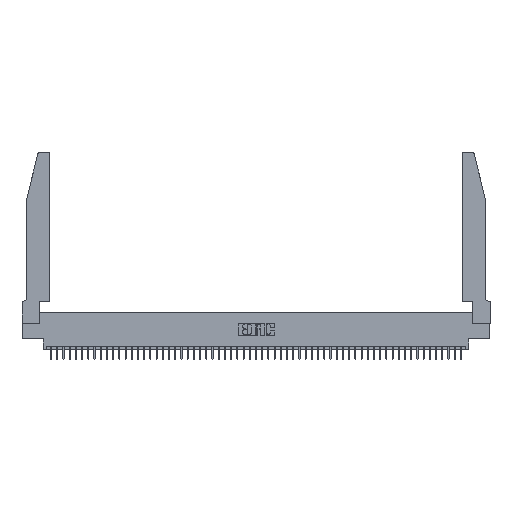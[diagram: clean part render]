
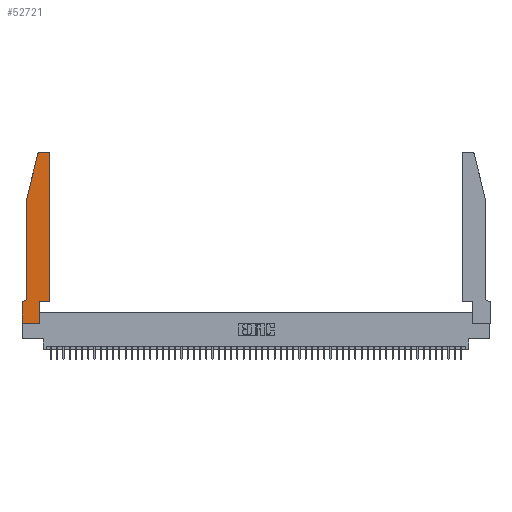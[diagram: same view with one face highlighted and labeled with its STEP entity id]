
A CAD part, top view. The second image highlights one B-rep face of the part: STEP entity #52721.
In plain terms, the highlighted planar face has unit normal (0, 0, 1).
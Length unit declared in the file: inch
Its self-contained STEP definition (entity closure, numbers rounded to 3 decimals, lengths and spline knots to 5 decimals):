
#729 = DIRECTION ( 'NONE',  ( 1., 0., 0. ) ) ;
#968 = VECTOR ( 'NONE', #33192, 39.37008 ) ;
#1160 = EDGE_CURVE ( 'NONE', #38254, #40192, #9611, .T. ) ;
#1197 = CARTESIAN_POINT ( 'NONE',  ( 0.4205, 2.72, 0.37 ) ) ;
#1478 = LINE ( 'NONE', #21008, #22473 ) ;
#1681 = LINE ( 'NONE', #25852, #3002 ) ;
#1808 = ORIENTED_EDGE ( 'NONE', *, *, #1160, .T. ) ;
#2245 = VERTEX_POINT ( 'NONE', #37265 ) ;
#2338 = DIRECTION ( 'NONE',  ( 0., 0., 1. ) ) ;
#2991 = CARTESIAN_POINT ( 'NONE',  ( 0.0055, 0.35, 0.37 ) ) ;
#3002 = VECTOR ( 'NONE', #729, 39.37008 ) ;
#3224 = ORIENTED_EDGE ( 'NONE', *, *, #48681, .T. ) ;
#4009 = CARTESIAN_POINT ( 'NONE',  ( 0.4205, 2.75, 0.37 ) ) ;
#5433 = DIRECTION ( 'NONE',  ( 1., 0., 0. ) ) ;
#7409 = ORIENTED_EDGE ( 'NONE', *, *, #41785, .T. ) ;
#7880 = CARTESIAN_POINT ( 'NONE',  ( 0., 0., 0.37 ) ) ;
#8603 = CARTESIAN_POINT ( 'NONE',  ( 0.4505, 2.72, 0.37 ) ) ;
#9611 = CIRCLE ( 'NONE', #31073, 0.03 ) ;
#10171 = VERTEX_POINT ( 'NONE', #50380 ) ;
#10530 = LINE ( 'NONE', #48544, #42684 ) ;
#10704 = CARTESIAN_POINT ( 'NONE',  ( 0.2865, 0., 0.37 ) ) ;
#10878 = DIRECTION ( 'NONE',  ( 0., 0., -1. ) ) ;
#11372 = CARTESIAN_POINT ( 'NONE',  ( 0., 0.35, 0.37 ) ) ;
#12225 = ORIENTED_EDGE ( 'NONE', *, *, #20809, .T. ) ;
#13235 = VERTEX_POINT ( 'NONE', #36837 ) ;
#14079 = ORIENTED_EDGE ( 'NONE', *, *, #31133, .T. ) ;
#14573 = VERTEX_POINT ( 'NONE', #11372 ) ;
#15166 = ORIENTED_EDGE ( 'NONE', *, *, #44168, .T. ) ;
#15667 = VERTEX_POINT ( 'NONE', #17763 ) ;
#15708 = VECTOR ( 'NONE', #51300, 39.37008 ) ;
#16157 = ORIENTED_EDGE ( 'NONE', *, *, #49384, .T. ) ;
#16404 = AXIS2_PLACEMENT_3D ( 'NONE', #36039, #10878, #40196 ) ;
#16542 = EDGE_CURVE ( 'NONE', #13235, #23261, #33527, .T. ) ;
#16600 = DIRECTION ( 'NONE',  ( -0.239, -0.971, 0. ) ) ;
#17763 = CARTESIAN_POINT ( 'NONE',  ( 0.25487, 2.72718, 0.37 ) ) ;
#17902 = CARTESIAN_POINT ( 'NONE',  ( 0.2605, 2.75, 0.37 ) ) ;
#17969 = VERTEX_POINT ( 'NONE', #10704 ) ;
#19285 = CARTESIAN_POINT ( 'NONE',  ( 0.2865, 0.35, 0.37 ) ) ;
#19625 = FACE_OUTER_BOUND ( 'NONE', #51829, .T. ) ;
#20610 = CARTESIAN_POINT ( 'NONE',  ( 0.0755, 2., 0.37 ) ) ;
#20809 = EDGE_CURVE ( 'NONE', #43978, #13235, #1478, .T. ) ;
#21008 = CARTESIAN_POINT ( 'NONE',  ( 0.0755, 2., 0.37 ) ) ;
#21282 = ORIENTED_EDGE ( 'NONE', *, *, #43305, .T. ) ;
#22114 = PLANE ( 'NONE',  #34845 ) ;
#22290 = CARTESIAN_POINT ( 'NONE',  ( 0., 0.35, 0.37 ) ) ;
#22473 = VECTOR ( 'NONE', #35866, 39.37008 ) ;
#23261 = VERTEX_POINT ( 'NONE', #2991 ) ;
#23272 = LINE ( 'NONE', #28945, #968 ) ;
#23498 = DIRECTION ( 'NONE',  ( 0., 1., 0. ) ) ;
#23555 = DIRECTION ( 'NONE',  ( 0., 1., 0. ) ) ;
#25852 = CARTESIAN_POINT ( 'NONE',  ( 0.4505, 0.35, 0.37 ) ) ;
#26543 = DIRECTION ( 'NONE',  ( 1., 0., 0. ) ) ;
#27492 = CARTESIAN_POINT ( 'NONE',  ( 0.284, 2.72, 0.37 ) ) ;
#27785 = CARTESIAN_POINT ( 'NONE',  ( 0.4505, 0.35, 0.37 ) ) ;
#28052 = VECTOR ( 'NONE', #44720, 39.37008 ) ;
#28945 = CARTESIAN_POINT ( 'NONE',  ( 0., 0., 0.37 ) ) ;
#30451 = EDGE_CURVE ( 'NONE', #17969, #2245, #31289, .T. ) ;
#30556 = DIRECTION ( 'NONE',  ( 0., 0., 1. ) ) ;
#30857 = EDGE_CURVE ( 'NONE', #2245, #10171, #1681, .T. ) ;
#31073 = AXIS2_PLACEMENT_3D ( 'NONE', #1197, #30556, #5433 ) ;
#31084 = VECTOR ( 'NONE', #16600, 39.37008 ) ;
#31133 = EDGE_CURVE ( 'NONE', #49515, #15667, #54010, .T. ) ;
#31289 = LINE ( 'NONE', #19285, #52131 ) ;
#31714 = DIRECTION ( 'NONE',  ( 1., 0., 0. ) ) ;
#31784 = LINE ( 'NONE', #27785, #52614 ) ;
#33192 = DIRECTION ( 'NONE',  ( 1., 0., 0. ) ) ;
#33527 = CIRCLE ( 'NONE', #16404, 0.07 ) ;
#34845 = AXIS2_PLACEMENT_3D ( 'NONE', #22290, #51516, #26543 ) ;
#35866 = DIRECTION ( 'NONE',  ( 0., -1., 0. ) ) ;
#36008 = DIRECTION ( 'NONE',  ( -1., 0., 0. ) ) ;
#36039 = CARTESIAN_POINT ( 'NONE',  ( 0.0055, 0.42, 0.37 ) ) ;
#36837 = CARTESIAN_POINT ( 'NONE',  ( 0.0755, 0.42, 0.37 ) ) ;
#37265 = CARTESIAN_POINT ( 'NONE',  ( 0.2865, 0.35, 0.37 ) ) ;
#38026 = LINE ( 'NONE', #17902, #15708 ) ;
#38231 = CARTESIAN_POINT ( 'NONE',  ( 0.284, 2.75, 0.37 ) ) ;
#38254 = VERTEX_POINT ( 'NONE', #8603 ) ;
#40192 = VERTEX_POINT ( 'NONE', #4009 ) ;
#40196 = DIRECTION ( 'NONE',  ( -1., 0., 0. ) ) ;
#40520 = CARTESIAN_POINT ( 'NONE',  ( 0., 0., 0.37 ) ) ;
#41785 = EDGE_CURVE ( 'NONE', #23261, #14573, #10530, .T. ) ;
#41856 = LINE ( 'NONE', #40520, #28052 ) ;
#42498 = VERTEX_POINT ( 'NONE', #7880 ) ;
#42684 = VECTOR ( 'NONE', #36008, 39.37008 ) ;
#43305 = EDGE_CURVE ( 'NONE', #40192, #49515, #38026, .T. ) ;
#43978 = VERTEX_POINT ( 'NONE', #47462 ) ;
#44168 = EDGE_CURVE ( 'NONE', #14573, #42498, #41856, .T. ) ;
#44720 = DIRECTION ( 'NONE',  ( 0., -1., 0. ) ) ;
#45160 = ORIENTED_EDGE ( 'NONE', *, *, #30451, .T. ) ;
#45873 = ORIENTED_EDGE ( 'NONE', *, *, #30857, .T. ) ;
#46787 = ORIENTED_EDGE ( 'NONE', *, *, #16542, .T. ) ;
#47462 = CARTESIAN_POINT ( 'NONE',  ( 0.0755, 2., 0.37 ) ) ;
#48544 = CARTESIAN_POINT ( 'NONE',  ( 0.0755, 0.35, 0.37 ) ) ;
#48681 = EDGE_CURVE ( 'NONE', #42498, #17969, #23272, .T. ) ;
#49014 = ORIENTED_EDGE ( 'NONE', *, *, #49165, .T. ) ;
#49165 = EDGE_CURVE ( 'NONE', #10171, #38254, #31784, .T. ) ;
#49384 = EDGE_CURVE ( 'NONE', #15667, #43978, #53226, .T. ) ;
#49515 = VERTEX_POINT ( 'NONE', #38231 ) ;
#50380 = CARTESIAN_POINT ( 'NONE',  ( 0.4505, 0.35, 0.37 ) ) ;
#51300 = DIRECTION ( 'NONE',  ( -1., 0., 0. ) ) ;
#51516 = DIRECTION ( 'NONE',  ( 0., 0., 1. ) ) ;
#51829 = EDGE_LOOP ( 'NONE', ( #21282, #14079, #16157, #12225, #46787, #7409, #15166, #3224, #45160, #45873, #49014, #1808 ) ) ;
#52131 = VECTOR ( 'NONE', #23498, 39.37008 ) ;
#52614 = VECTOR ( 'NONE', #23555, 39.37008 ) ;
#52721 = ADVANCED_FACE ( 'NONE', ( #19625 ), #22114, .T. ) ;
#53226 = LINE ( 'NONE', #20610, #31084 ) ;
#53902 = AXIS2_PLACEMENT_3D ( 'NONE', #27492, #2338, #31714 ) ;
#54010 = CIRCLE ( 'NONE', #53902, 0.03 ) ;
